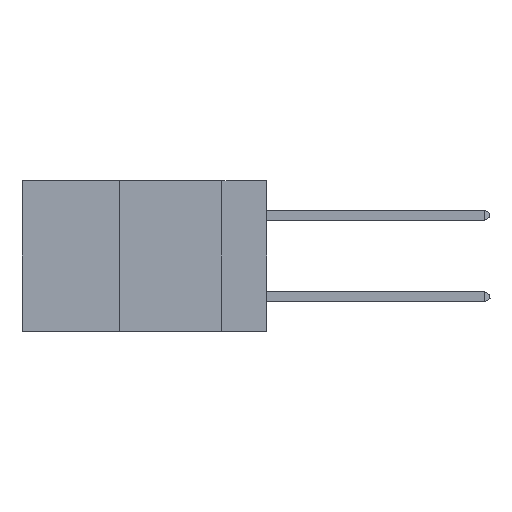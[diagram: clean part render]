
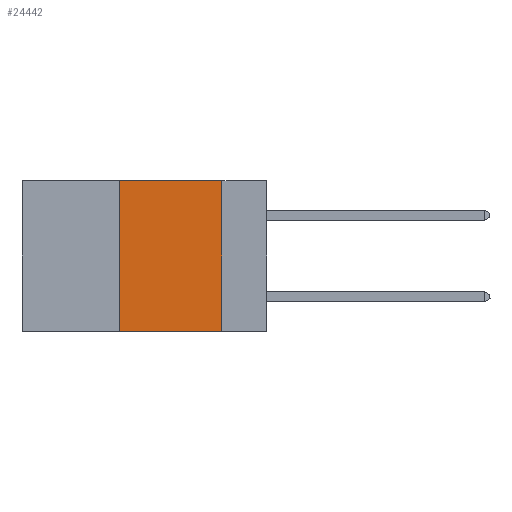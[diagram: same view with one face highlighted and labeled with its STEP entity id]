
A CAD part, left-side view. The second image highlights one B-rep face of the part: STEP entity #24442.
In plain terms, the highlighted planar face has unit normal (-1, 0, 0).
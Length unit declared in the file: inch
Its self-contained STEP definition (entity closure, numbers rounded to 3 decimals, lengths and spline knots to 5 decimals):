
#24 = DIRECTION ( 'NONE',  ( 0., -1., 0. ) ) ;
#159 = DIRECTION ( 'NONE',  ( 0., -1., 0. ) ) ;
#707 = EDGE_CURVE ( 'NONE', #1668, #2139, #12673, .T. ) ;
#709 = VECTOR ( 'NONE', #24, 39.37008 ) ;
#919 = AXIS2_PLACEMENT_3D ( 'NONE', #16727, #5007, #12996 ) ;
#1191 = EDGE_CURVE ( 'NONE', #12433, #21763, #10823, .T. ) ;
#1225 = DIRECTION ( 'NONE',  ( 0., 0., 1. ) ) ;
#1668 = VERTEX_POINT ( 'NONE', #6687 ) ;
#2002 = CARTESIAN_POINT ( 'NONE',  ( 0., 0.6, 0. ) ) ;
#2139 = VERTEX_POINT ( 'NONE', #21012 ) ;
#3144 = PLANE ( 'NONE',  #919 ) ;
#5007 = DIRECTION ( 'NONE',  ( 1., 0., 0. ) ) ;
#5333 = LINE ( 'NONE', #24017, #18750 ) ;
#6095 = EDGE_CURVE ( 'NONE', #12433, #1668, #5333, .T. ) ;
#6253 = VECTOR ( 'NONE', #159, 39.37008 ) ;
#6687 = CARTESIAN_POINT ( 'NONE',  ( 0., 0.36, 0. ) ) ;
#6799 = ORIENTED_EDGE ( 'NONE', *, *, #1191, .T. ) ;
#8757 = CARTESIAN_POINT ( 'NONE',  ( 0., 0.6, -0.37 ) ) ;
#9863 = EDGE_LOOP ( 'NONE', ( #21745, #24561, #14544, #6799 ) ) ;
#10823 = LINE ( 'NONE', #8757, #709 ) ;
#11175 = DIRECTION ( 'NONE',  ( 0., 0., -1. ) ) ;
#12433 = VERTEX_POINT ( 'NONE', #23159 ) ;
#12673 = LINE ( 'NONE', #2002, #6253 ) ;
#12879 = LINE ( 'NONE', #24914, #17435 ) ;
#12996 = DIRECTION ( 'NONE',  ( 0., 0., -1. ) ) ;
#14544 = ORIENTED_EDGE ( 'NONE', *, *, #6095, .F. ) ;
#16727 = CARTESIAN_POINT ( 'NONE',  ( 0., 0.6, 0. ) ) ;
#17435 = VECTOR ( 'NONE', #11175, 39.37008 ) ;
#18750 = VECTOR ( 'NONE', #1225, 39.37008 ) ;
#19656 = FACE_OUTER_BOUND ( 'NONE', #9863, .T. ) ;
#20581 = EDGE_CURVE ( 'NONE', #2139, #21763, #12879, .T. ) ;
#21012 = CARTESIAN_POINT ( 'NONE',  ( 0., 0.11, 0. ) ) ;
#21745 = ORIENTED_EDGE ( 'NONE', *, *, #20581, .F. ) ;
#21763 = VERTEX_POINT ( 'NONE', #23046 ) ;
#23046 = CARTESIAN_POINT ( 'NONE',  ( 0., 0.11, -0.37 ) ) ;
#23159 = CARTESIAN_POINT ( 'NONE',  ( 0., 0.36, -0.37 ) ) ;
#24017 = CARTESIAN_POINT ( 'NONE',  ( 0., 0.36, 0. ) ) ;
#24442 = ADVANCED_FACE ( 'NONE', ( #19656 ), #3144, .F. ) ;
#24561 = ORIENTED_EDGE ( 'NONE', *, *, #707, .F. ) ;
#24914 = CARTESIAN_POINT ( 'NONE',  ( 0., 0.11, 0. ) ) ;
